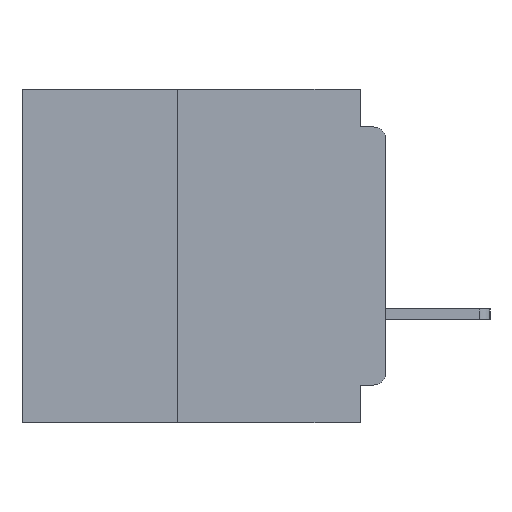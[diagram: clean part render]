
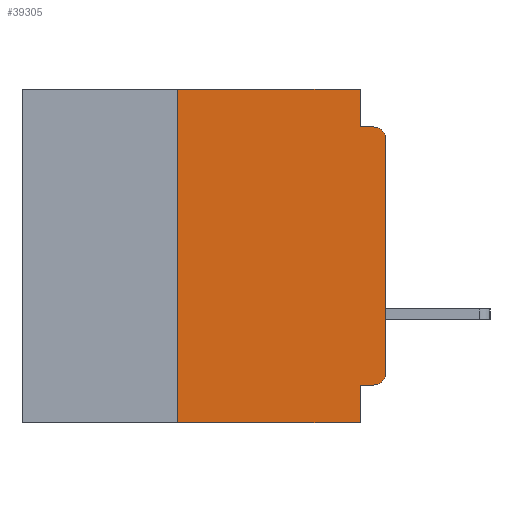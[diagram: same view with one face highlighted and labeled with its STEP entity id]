
A CAD part, left-side view. The second image highlights one B-rep face of the part: STEP entity #39305.
In plain terms, the highlighted planar face has unit normal (-1, 0, 0).
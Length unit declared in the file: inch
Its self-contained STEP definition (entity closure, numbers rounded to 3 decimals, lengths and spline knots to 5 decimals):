
#1541 = CARTESIAN_POINT ( 'NONE',  ( 0., 0.437, 0. ) ) ;
#1688 = CARTESIAN_POINT ( 'NONE',  ( 0., 0., 0. ) ) ;
#3721 = CARTESIAN_POINT ( 'NONE',  ( 0., 0.031, -0.4 ) ) ;
#3980 = DIRECTION ( 'NONE',  ( 0., 0., -1. ) ) ;
#5345 = CARTESIAN_POINT ( 'NONE',  ( 0., 0.25, 0. ) ) ;
#5940 = CARTESIAN_POINT ( 'NONE',  ( 0., 0.437, 0. ) ) ;
#6238 = CARTESIAN_POINT ( 'NONE',  ( 0., 0.015, -0.355 ) ) ;
#6464 = EDGE_CURVE ( 'NONE', #52167, #18420, #39086, .T. ) ;
#7645 = VECTOR ( 'NONE', #22490, 39.37008 ) ;
#9455 = CARTESIAN_POINT ( 'NONE',  ( 0., 0.031, -0.355 ) ) ;
#10097 = EDGE_CURVE ( 'NONE', #51204, #27855, #21143, .T. ) ;
#10261 = VECTOR ( 'NONE', #16122, 39.37008 ) ;
#10508 = ORIENTED_EDGE ( 'NONE', *, *, #6464, .F. ) ;
#11024 = LINE ( 'NONE', #19098, #42072 ) ;
#11233 = ORIENTED_EDGE ( 'NONE', *, *, #17337, .F. ) ;
#11558 = LINE ( 'NONE', #40314, #10261 ) ;
#12280 = CARTESIAN_POINT ( 'NONE',  ( 0., 0., -0.06 ) ) ;
#12497 = DIRECTION ( 'NONE',  ( 0., 1., 0. ) ) ;
#12737 = VERTEX_POINT ( 'NONE', #26387 ) ;
#13211 = CIRCLE ( 'NONE', #31858, 0.015 ) ;
#13938 = DIRECTION ( 'NONE',  ( 0., 0., 1. ) ) ;
#13970 = PLANE ( 'NONE',  #36764 ) ;
#14027 = CARTESIAN_POINT ( 'NONE',  ( 0., 0.031, -0.045 ) ) ;
#14743 = EDGE_CURVE ( 'NONE', #19574, #24584, #11558, .T. ) ;
#16122 = DIRECTION ( 'NONE',  ( 0., 0., -1. ) ) ;
#16316 = VECTOR ( 'NONE', #23526, 39.37008 ) ;
#16340 = EDGE_CURVE ( 'NONE', #27709, #42207, #51303, .T. ) ;
#16456 = DIRECTION ( 'NONE',  ( -1., 0., 0. ) ) ;
#16655 = EDGE_CURVE ( 'NONE', #51204, #27709, #13211, .T. ) ;
#17337 = EDGE_CURVE ( 'NONE', #24584, #12737, #32885, .T. ) ;
#17623 = DIRECTION ( 'NONE',  ( 0., -1., 0. ) ) ;
#18232 = CARTESIAN_POINT ( 'NONE',  ( 0., 0.437, -0.4 ) ) ;
#18420 = VERTEX_POINT ( 'NONE', #5345 ) ;
#19098 = CARTESIAN_POINT ( 'NONE',  ( 0., 0.031, -0.4 ) ) ;
#19574 = VERTEX_POINT ( 'NONE', #25658 ) ;
#21143 = LINE ( 'NONE', #36829, #42621 ) ;
#21619 = ORIENTED_EDGE ( 'NONE', *, *, #38724, .F. ) ;
#22196 = DIRECTION ( 'NONE',  ( 1., 0., 0. ) ) ;
#22490 = DIRECTION ( 'NONE',  ( 0., -1., 0. ) ) ;
#23526 = DIRECTION ( 'NONE',  ( 0., 0., 1. ) ) ;
#23908 = ORIENTED_EDGE ( 'NONE', *, *, #30222, .T. ) ;
#24584 = VERTEX_POINT ( 'NONE', #14027 ) ;
#24870 = CARTESIAN_POINT ( 'NONE',  ( 0., 0., -0.34 ) ) ;
#25658 = CARTESIAN_POINT ( 'NONE',  ( 0., 0.031, 0. ) ) ;
#26387 = CARTESIAN_POINT ( 'NONE',  ( 0., 0.015, -0.045 ) ) ;
#27611 = VECTOR ( 'NONE', #42371, 39.37008 ) ;
#27709 = VERTEX_POINT ( 'NONE', #24870 ) ;
#27855 = VERTEX_POINT ( 'NONE', #9455 ) ;
#28463 = DIRECTION ( 'NONE',  ( -1., 0., 0. ) ) ;
#28492 = ORIENTED_EDGE ( 'NONE', *, *, #16340, .T. ) ;
#28578 = ORIENTED_EDGE ( 'NONE', *, *, #34767, .F. ) ;
#30222 = EDGE_CURVE ( 'NONE', #42207, #12737, #38318, .T. ) ;
#31540 = ORIENTED_EDGE ( 'NONE', *, *, #14743, .F. ) ;
#31858 = AXIS2_PLACEMENT_3D ( 'NONE', #40657, #16456, #44725 ) ;
#32885 = LINE ( 'NONE', #41629, #42304 ) ;
#34767 = EDGE_CURVE ( 'NONE', #27855, #47903, #11024, .T. ) ;
#36746 = ORIENTED_EDGE ( 'NONE', *, *, #10097, .F. ) ;
#36764 = AXIS2_PLACEMENT_3D ( 'NONE', #1541, #22196, #50443 ) ;
#36829 = CARTESIAN_POINT ( 'NONE',  ( 0., 0., -0.355 ) ) ;
#37169 = ORIENTED_EDGE ( 'NONE', *, *, #40156, .T. ) ;
#38318 = CIRCLE ( 'NONE', #44135, 0.015 ) ;
#38724 = EDGE_CURVE ( 'NONE', #18420, #19574, #46536, .T. ) ;
#38974 = CARTESIAN_POINT ( 'NONE',  ( 0., 0.25, -0.4 ) ) ;
#39086 = LINE ( 'NONE', #51765, #16316 ) ;
#39305 = ADVANCED_FACE ( 'NONE', ( #52173 ), #13970, .F. ) ;
#40049 = LINE ( 'NONE', #18232, #7645 ) ;
#40156 = EDGE_CURVE ( 'NONE', #52167, #47903, #40049, .T. ) ;
#40314 = CARTESIAN_POINT ( 'NONE',  ( 0., 0.031, 0. ) ) ;
#40657 = CARTESIAN_POINT ( 'NONE',  ( 0., 0.015, -0.34 ) ) ;
#41629 = CARTESIAN_POINT ( 'NONE',  ( 0., 0., -0.045 ) ) ;
#42072 = VECTOR ( 'NONE', #51229, 39.37008 ) ;
#42207 = VERTEX_POINT ( 'NONE', #12280 ) ;
#42304 = VECTOR ( 'NONE', #17623, 39.37008 ) ;
#42371 = DIRECTION ( 'NONE',  ( 0., -1., 0. ) ) ;
#42621 = VECTOR ( 'NONE', #12497, 39.37008 ) ;
#42675 = EDGE_LOOP ( 'NONE', ( #28492, #23908, #11233, #31540, #21619, #10508, #37169, #28578, #36746, #45501 ) ) ;
#44135 = AXIS2_PLACEMENT_3D ( 'NONE', #52656, #28463, #3980 ) ;
#44725 = DIRECTION ( 'NONE',  ( 0., 0., -1. ) ) ;
#45501 = ORIENTED_EDGE ( 'NONE', *, *, #16655, .T. ) ;
#46536 = LINE ( 'NONE', #5940, #27611 ) ;
#47903 = VERTEX_POINT ( 'NONE', #3721 ) ;
#48770 = VECTOR ( 'NONE', #13938, 39.37008 ) ;
#50443 = DIRECTION ( 'NONE',  ( 0., 0., -1. ) ) ;
#51204 = VERTEX_POINT ( 'NONE', #6238 ) ;
#51229 = DIRECTION ( 'NONE',  ( 0., 0., -1. ) ) ;
#51303 = LINE ( 'NONE', #1688, #48770 ) ;
#51765 = CARTESIAN_POINT ( 'NONE',  ( 0., 0.25, -0.4 ) ) ;
#52167 = VERTEX_POINT ( 'NONE', #38974 ) ;
#52173 = FACE_OUTER_BOUND ( 'NONE', #42675, .T. ) ;
#52656 = CARTESIAN_POINT ( 'NONE',  ( 0., 0.015, -0.06 ) ) ;
